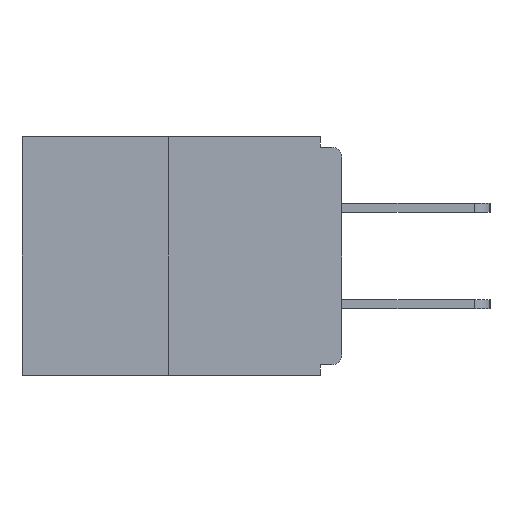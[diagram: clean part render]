
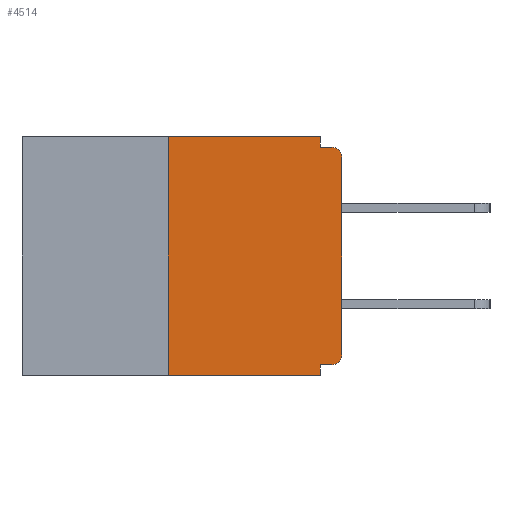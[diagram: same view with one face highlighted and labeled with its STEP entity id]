
A CAD part, left-side view. The second image highlights one B-rep face of the part: STEP entity #4514.
In plain terms, the highlighted planar face has unit normal (-1, 0, 0).
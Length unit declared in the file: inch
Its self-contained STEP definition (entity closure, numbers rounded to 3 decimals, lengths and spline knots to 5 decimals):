
#55 = ORIENTED_EDGE ( 'NONE', *, *, #4055, .F. ) ;
#208 = ORIENTED_EDGE ( 'NONE', *, *, #10927, .T. ) ;
#309 = ORIENTED_EDGE ( 'NONE', *, *, #13283, .F. ) ;
#322 = EDGE_CURVE ( 'NONE', #1316, #2838, #8216, .T. ) ;
#374 = EDGE_CURVE ( 'NONE', #8893, #11791, #6285, .T. ) ;
#691 = LINE ( 'NONE', #8324, #5317 ) ;
#698 = ORIENTED_EDGE ( 'NONE', *, *, #374, .F. ) ;
#771 = EDGE_CURVE ( 'NONE', #11514, #4637, #11007, .T. ) ;
#773 = EDGE_CURVE ( 'NONE', #11791, #2061, #10485, .T. ) ;
#780 = DIRECTION ( 'NONE',  ( 0., 0., -1. ) ) ;
#825 = PLANE ( 'NONE',  #6832 ) ;
#1316 = VERTEX_POINT ( 'NONE', #4838 ) ;
#1884 = ORIENTED_EDGE ( 'NONE', *, *, #771, .F. ) ;
#1966 = DIRECTION ( 'NONE',  ( 1., 0., 0. ) ) ;
#2061 = VERTEX_POINT ( 'NONE', #12267 ) ;
#2287 = EDGE_CURVE ( 'NONE', #3376, #11514, #691, .T. ) ;
#2418 = ORIENTED_EDGE ( 'NONE', *, *, #2287, .F. ) ;
#2496 = VECTOR ( 'NONE', #5870, 39.37008 ) ;
#2576 = VECTOR ( 'NONE', #8490, 39.37008 ) ;
#2838 = VERTEX_POINT ( 'NONE', #6923 ) ;
#3032 = DIRECTION ( 'NONE',  ( 0., 0., -1. ) ) ;
#3356 = DIRECTION ( 'NONE',  ( 0., -1., 0. ) ) ;
#3376 = VERTEX_POINT ( 'NONE', #4507 ) ;
#3584 = CARTESIAN_POINT ( 'NONE',  ( 0., 0.015, -0.313 ) ) ;
#3691 = CARTESIAN_POINT ( 'NONE',  ( 0., 0., -0.313 ) ) ;
#3704 = CARTESIAN_POINT ( 'NONE',  ( 0., 0.46, -0.343 ) ) ;
#4042 = EDGE_CURVE ( 'NONE', #9148, #1316, #11080, .T. ) ;
#4055 = EDGE_CURVE ( 'NONE', #14304, #2838, #10737, .T. ) ;
#4152 = CARTESIAN_POINT ( 'NONE',  ( 0., 0.25, -0.343 ) ) ;
#4384 = AXIS2_PLACEMENT_3D ( 'NONE', #13162, #10853, #780 ) ;
#4507 = CARTESIAN_POINT ( 'NONE',  ( 0., 0.015, -0.328 ) ) ;
#4514 = ADVANCED_FACE ( 'NONE', ( #6679 ), #825, .F. ) ;
#4637 = VERTEX_POINT ( 'NONE', #10631 ) ;
#4705 = DIRECTION ( 'NONE',  ( -1., 0., 0. ) ) ;
#4838 = CARTESIAN_POINT ( 'NONE',  ( 0., 0., -0.03 ) ) ;
#5056 = CARTESIAN_POINT ( 'NONE',  ( 0., 0.46, 0. ) ) ;
#5216 = VECTOR ( 'NONE', #12945, 39.37008 ) ;
#5231 = VECTOR ( 'NONE', #14502, 39.37008 ) ;
#5317 = VECTOR ( 'NONE', #7093, 39.37008 ) ;
#5524 = DIRECTION ( 'NONE',  ( 0., 0., 1. ) ) ;
#5671 = CARTESIAN_POINT ( 'NONE',  ( 0., 0., 0. ) ) ;
#5845 = DIRECTION ( 'NONE',  ( 0., 0., -1. ) ) ;
#5857 = CIRCLE ( 'NONE', #6163, 0.015 ) ;
#5870 = DIRECTION ( 'NONE',  ( 0., -1., 0. ) ) ;
#6163 = AXIS2_PLACEMENT_3D ( 'NONE', #3584, #4705, #5845 ) ;
#6285 = LINE ( 'NONE', #6590, #6982 ) ;
#6365 = ORIENTED_EDGE ( 'NONE', *, *, #4042, .T. ) ;
#6387 = CARTESIAN_POINT ( 'NONE',  ( 0., 0.46, 0. ) ) ;
#6582 = ORIENTED_EDGE ( 'NONE', *, *, #10528, .T. ) ;
#6590 = CARTESIAN_POINT ( 'NONE',  ( 0., 0.25, 0. ) ) ;
#6636 = ORIENTED_EDGE ( 'NONE', *, *, #322, .T. ) ;
#6679 = FACE_OUTER_BOUND ( 'NONE', #7162, .T. ) ;
#6832 = AXIS2_PLACEMENT_3D ( 'NONE', #6387, #1966, #3032 ) ;
#6923 = CARTESIAN_POINT ( 'NONE',  ( 0., 0.015, -0.015 ) ) ;
#6982 = VECTOR ( 'NONE', #13450, 39.37008 ) ;
#7093 = DIRECTION ( 'NONE',  ( 0., 1., 0. ) ) ;
#7162 = EDGE_LOOP ( 'NONE', ( #10656, #698, #6582, #1884, #2418, #208, #6365, #6636, #55, #309 ) ) ;
#8216 = CIRCLE ( 'NONE', #4384, 0.015 ) ;
#8324 = CARTESIAN_POINT ( 'NONE',  ( 0., 0., -0.328 ) ) ;
#8418 = LINE ( 'NONE', #14456, #5231 ) ;
#8490 = DIRECTION ( 'NONE',  ( 0., -1., 0. ) ) ;
#8893 = VERTEX_POINT ( 'NONE', #4152 ) ;
#9148 = VERTEX_POINT ( 'NONE', #3691 ) ;
#9670 = VECTOR ( 'NONE', #3356, 39.37008 ) ;
#9921 = LINE ( 'NONE', #3704, #2496 ) ;
#10485 = LINE ( 'NONE', #5056, #2576 ) ;
#10491 = CARTESIAN_POINT ( 'NONE',  ( 0., 0.25, 0. ) ) ;
#10528 = EDGE_CURVE ( 'NONE', #8893, #4637, #9921, .T. ) ;
#10631 = CARTESIAN_POINT ( 'NONE',  ( 0., 0.031, -0.343 ) ) ;
#10656 = ORIENTED_EDGE ( 'NONE', *, *, #773, .F. ) ;
#10737 = LINE ( 'NONE', #13333, #9670 ) ;
#10853 = DIRECTION ( 'NONE',  ( -1., 0., 0. ) ) ;
#10927 = EDGE_CURVE ( 'NONE', #3376, #9148, #5857, .T. ) ;
#11007 = LINE ( 'NONE', #13043, #5216 ) ;
#11080 = LINE ( 'NONE', #5671, #11600 ) ;
#11514 = VERTEX_POINT ( 'NONE', #13159 ) ;
#11600 = VECTOR ( 'NONE', #5524, 39.37008 ) ;
#11791 = VERTEX_POINT ( 'NONE', #10491 ) ;
#12267 = CARTESIAN_POINT ( 'NONE',  ( 0., 0.031, 0. ) ) ;
#12945 = DIRECTION ( 'NONE',  ( 0., 0., -1. ) ) ;
#13043 = CARTESIAN_POINT ( 'NONE',  ( 0., 0.031, -0.343 ) ) ;
#13159 = CARTESIAN_POINT ( 'NONE',  ( 0., 0.031, -0.328 ) ) ;
#13162 = CARTESIAN_POINT ( 'NONE',  ( 0., 0.015, -0.03 ) ) ;
#13283 = EDGE_CURVE ( 'NONE', #2061, #14304, #8418, .T. ) ;
#13333 = CARTESIAN_POINT ( 'NONE',  ( 0., 0., -0.015 ) ) ;
#13450 = DIRECTION ( 'NONE',  ( 0., 0., 1. ) ) ;
#13935 = CARTESIAN_POINT ( 'NONE',  ( 0., 0.031, -0.015 ) ) ;
#14304 = VERTEX_POINT ( 'NONE', #13935 ) ;
#14456 = CARTESIAN_POINT ( 'NONE',  ( 0., 0.031, 0. ) ) ;
#14502 = DIRECTION ( 'NONE',  ( 0., 0., -1. ) ) ;
